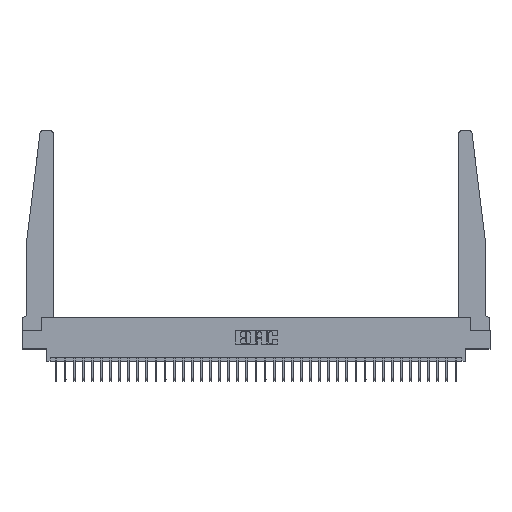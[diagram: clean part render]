
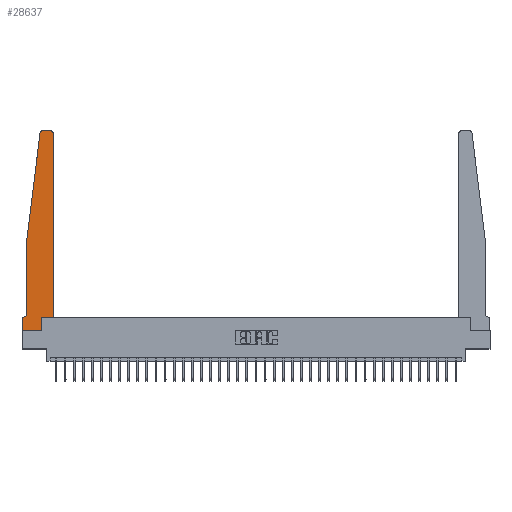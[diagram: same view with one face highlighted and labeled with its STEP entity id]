
A CAD part, top view. The second image highlights one B-rep face of the part: STEP entity #28637.
In plain terms, the highlighted planar face has unit normal (0, 0, 1).
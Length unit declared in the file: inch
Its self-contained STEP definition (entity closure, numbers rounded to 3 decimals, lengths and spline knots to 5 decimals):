
#603 = EDGE_CURVE ( 'NONE', #24675, #7251, #3570, .T. ) ;
#709 = EDGE_CURVE ( 'NONE', #23010, #5758, #9253, .T. ) ;
#1759 = CARTESIAN_POINT ( 'NONE',  ( 0.2605, 0.18, 0.37 ) ) ;
#1877 = ORIENTED_EDGE ( 'NONE', *, *, #19846, .T. ) ;
#2036 = CARTESIAN_POINT ( 'NONE',  ( 0.395, 2.72, 0.37 ) ) ;
#2250 = CIRCLE ( 'NONE', #30981, 0.05 ) ;
#2355 = CARTESIAN_POINT ( 'NONE',  ( 0.27653, 2.75, 0.37 ) ) ;
#2606 = DIRECTION ( 'NONE',  ( 0., 0., 1. ) ) ;
#3254 = DIRECTION ( 'NONE',  ( -1., 0., 0. ) ) ;
#3570 = LINE ( 'NONE', #16339, #23846 ) ;
#4666 = CARTESIAN_POINT ( 'NONE',  ( 0.065, 1.25, 0.37 ) ) ;
#4774 = CARTESIAN_POINT ( 'NONE',  ( 0.27653, 2.72, 0.37 ) ) ;
#5684 = CARTESIAN_POINT ( 'NONE',  ( 0., 0.1875, 0.37 ) ) ;
#5758 = VERTEX_POINT ( 'NONE', #11658 ) ;
#5819 = DIRECTION ( 'NONE',  ( 0., -1., 0. ) ) ;
#5834 = VERTEX_POINT ( 'NONE', #4666 ) ;
#5860 = LINE ( 'NONE', #21152, #22466 ) ;
#6326 = CARTESIAN_POINT ( 'NONE',  ( 0.065, 0.2375, 0.37 ) ) ;
#6608 = AXIS2_PLACEMENT_3D ( 'NONE', #2036, #19134, #24501 ) ;
#6942 = CARTESIAN_POINT ( 'NONE',  ( 0., 0.1875, 0.37 ) ) ;
#7251 = VERTEX_POINT ( 'NONE', #20611 ) ;
#7615 = ORIENTED_EDGE ( 'NONE', *, *, #13778, .T. ) ;
#7783 = CARTESIAN_POINT ( 'NONE',  ( 0., 0., 0.37 ) ) ;
#8904 = LINE ( 'NONE', #21052, #24374 ) ;
#9004 = ORIENTED_EDGE ( 'NONE', *, *, #16619, .T. ) ;
#9052 = EDGE_CURVE ( 'NONE', #5834, #25851, #14265, .T. ) ;
#9253 = CIRCLE ( 'NONE', #6608, 0.03 ) ;
#10045 = CARTESIAN_POINT ( 'NONE',  ( 0.065, 0.1875, 0.37 ) ) ;
#10297 = VERTEX_POINT ( 'NONE', #2355 ) ;
#10382 = VECTOR ( 'NONE', #5819, 39.37008 ) ;
#10470 = VECTOR ( 'NONE', #12214, 39.37008 ) ;
#11223 = CARTESIAN_POINT ( 'NONE',  ( 0.2605, 0., 0.37 ) ) ;
#11267 = DIRECTION ( 'NONE',  ( 0., 0., -1. ) ) ;
#11377 = ORIENTED_EDGE ( 'NONE', *, *, #9052, .T. ) ;
#11416 = ORIENTED_EDGE ( 'NONE', *, *, #18290, .T. ) ;
#11658 = CARTESIAN_POINT ( 'NONE',  ( 0.395, 2.75, 0.37 ) ) ;
#11756 = DIRECTION ( 'NONE',  ( 0., 1., 0. ) ) ;
#12214 = DIRECTION ( 'NONE',  ( -1., 0., 0. ) ) ;
#13731 = AXIS2_PLACEMENT_3D ( 'NONE', #5684, #15794, #22651 ) ;
#13778 = EDGE_CURVE ( 'NONE', #25851, #18237, #2250, .T. ) ;
#14265 = LINE ( 'NONE', #28930, #21930 ) ;
#14889 = ORIENTED_EDGE ( 'NONE', *, *, #30930, .T. ) ;
#15055 = DIRECTION ( 'NONE',  ( 1., 0., 0. ) ) ;
#15085 = CARTESIAN_POINT ( 'NONE',  ( 0.2605, 0.18, 0.37 ) ) ;
#15794 = DIRECTION ( 'NONE',  ( 0., 0., 1. ) ) ;
#16339 = CARTESIAN_POINT ( 'NONE',  ( 0.425, 0.18, 0.37 ) ) ;
#16487 = ORIENTED_EDGE ( 'NONE', *, *, #30108, .T. ) ;
#16619 = EDGE_CURVE ( 'NONE', #19235, #19446, #20607, .T. ) ;
#17166 = ORIENTED_EDGE ( 'NONE', *, *, #29461, .T. ) ;
#17581 = ORIENTED_EDGE ( 'NONE', *, *, #709, .T. ) ;
#18237 = VERTEX_POINT ( 'NONE', #30587 ) ;
#18290 = EDGE_CURVE ( 'NONE', #10297, #30334, #26352, .T. ) ;
#19134 = DIRECTION ( 'NONE',  ( 0., 0., 1. ) ) ;
#19235 = VERTEX_POINT ( 'NONE', #6942 ) ;
#19446 = VERTEX_POINT ( 'NONE', #7783 ) ;
#19846 = EDGE_CURVE ( 'NONE', #18237, #19235, #25193, .T. ) ;
#20058 = DIRECTION ( 'NONE',  ( -0.122, -0.992, 0. ) ) ;
#20371 = CARTESIAN_POINT ( 'NONE',  ( 0.065, 1.25, 0.37 ) ) ;
#20461 = PLANE ( 'NONE',  #13731 ) ;
#20553 = LINE ( 'NONE', #20371, #29744 ) ;
#20607 = LINE ( 'NONE', #20917, #10382 ) ;
#20611 = CARTESIAN_POINT ( 'NONE',  ( 0.425, 0.18, 0.37 ) ) ;
#20679 = CARTESIAN_POINT ( 'NONE',  ( 0.425, 0.18, 0.37 ) ) ;
#20917 = CARTESIAN_POINT ( 'NONE',  ( 0., 0., 0.37 ) ) ;
#21052 = CARTESIAN_POINT ( 'NONE',  ( 0.25, 2.75, 0.37 ) ) ;
#21152 = CARTESIAN_POINT ( 'NONE',  ( 0., 0., 0.37 ) ) ;
#21414 = DIRECTION ( 'NONE',  ( -1., 0., 0. ) ) ;
#21890 = DIRECTION ( 'NONE',  ( 0., -1., 0. ) ) ;
#21930 = VECTOR ( 'NONE', #21890, 39.37008 ) ;
#22466 = VECTOR ( 'NONE', #31356, 39.37008 ) ;
#22651 = DIRECTION ( 'NONE',  ( 1., 0., 0. ) ) ;
#23010 = VERTEX_POINT ( 'NONE', #27604 ) ;
#23194 = DIRECTION ( 'NONE',  ( 0., 1., 0. ) ) ;
#23295 = VECTOR ( 'NONE', #23194, 39.37008 ) ;
#23846 = VECTOR ( 'NONE', #24178, 39.37008 ) ;
#24178 = DIRECTION ( 'NONE',  ( 1., 0., 0. ) ) ;
#24374 = VECTOR ( 'NONE', #3254, 39.37008 ) ;
#24493 = CARTESIAN_POINT ( 'NONE',  ( 0.24675, 2.72367, 0.37 ) ) ;
#24501 = DIRECTION ( 'NONE',  ( 1., 0., 0. ) ) ;
#24675 = VERTEX_POINT ( 'NONE', #15085 ) ;
#24735 = AXIS2_PLACEMENT_3D ( 'NONE', #4774, #2606, #15055 ) ;
#25057 = ORIENTED_EDGE ( 'NONE', *, *, #29379, .T. ) ;
#25193 = LINE ( 'NONE', #10045, #10470 ) ;
#25851 = VERTEX_POINT ( 'NONE', #6326 ) ;
#26265 = CARTESIAN_POINT ( 'NONE',  ( 0.015, 0.2375, 0.37 ) ) ;
#26352 = CIRCLE ( 'NONE', #24735, 0.03 ) ;
#27604 = CARTESIAN_POINT ( 'NONE',  ( 0.425, 2.72, 0.37 ) ) ;
#27789 = ORIENTED_EDGE ( 'NONE', *, *, #32584, .T. ) ;
#28149 = VECTOR ( 'NONE', #11756, 39.37008 ) ;
#28359 = ORIENTED_EDGE ( 'NONE', *, *, #603, .T. ) ;
#28368 = VERTEX_POINT ( 'NONE', #11223 ) ;
#28499 = FACE_OUTER_BOUND ( 'NONE', #30519, .T. ) ;
#28637 = ADVANCED_FACE ( 'NONE', ( #28499 ), #20461, .T. ) ;
#28930 = CARTESIAN_POINT ( 'NONE',  ( 0.065, 1.25, 0.37 ) ) ;
#29379 = EDGE_CURVE ( 'NONE', #28368, #24675, #29930, .T. ) ;
#29461 = EDGE_CURVE ( 'NONE', #30334, #5834, #20553, .T. ) ;
#29744 = VECTOR ( 'NONE', #20058, 39.37008 ) ;
#29930 = LINE ( 'NONE', #1759, #28149 ) ;
#30108 = EDGE_CURVE ( 'NONE', #7251, #23010, #31520, .T. ) ;
#30334 = VERTEX_POINT ( 'NONE', #24493 ) ;
#30519 = EDGE_LOOP ( 'NONE', ( #14889, #11416, #17166, #11377, #7615, #1877, #9004, #27789, #25057, #28359, #16487, #17581 ) ) ;
#30587 = CARTESIAN_POINT ( 'NONE',  ( 0.015, 0.1875, 0.37 ) ) ;
#30930 = EDGE_CURVE ( 'NONE', #5758, #10297, #8904, .T. ) ;
#30981 = AXIS2_PLACEMENT_3D ( 'NONE', #26265, #11267, #21414 ) ;
#31356 = DIRECTION ( 'NONE',  ( 1., 0., 0. ) ) ;
#31520 = LINE ( 'NONE', #20679, #23295 ) ;
#32584 = EDGE_CURVE ( 'NONE', #19446, #28368, #5860, .T. ) ;
